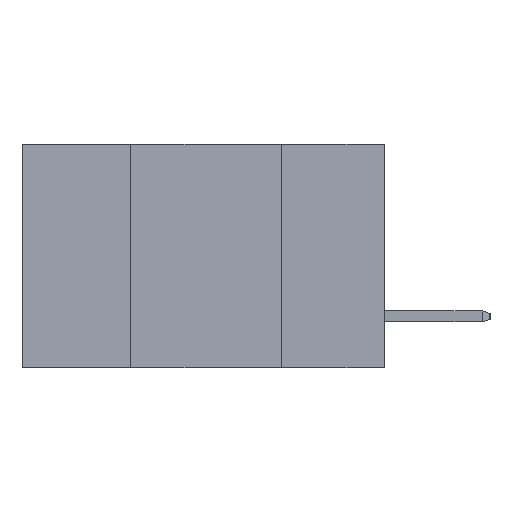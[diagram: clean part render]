
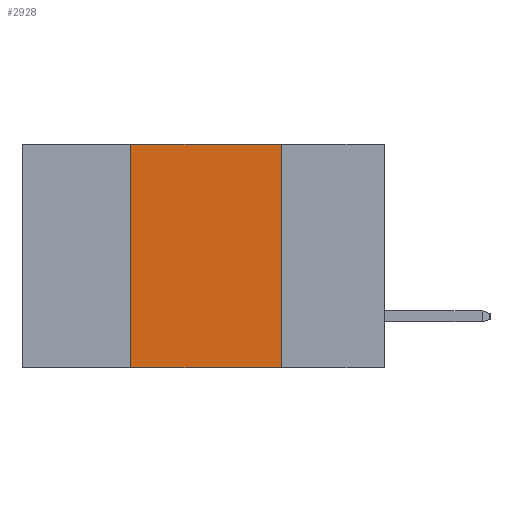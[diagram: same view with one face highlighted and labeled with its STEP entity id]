
A CAD part, left-side view. The second image highlights one B-rep face of the part: STEP entity #2928.
In plain terms, the highlighted planar face has unit normal (-1, 0, 0).
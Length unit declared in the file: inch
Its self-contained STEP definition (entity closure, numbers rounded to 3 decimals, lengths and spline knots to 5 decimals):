
#349 = ORIENTED_EDGE ( 'NONE', *, *, #1069, .F. ) ;
#1027 = LINE ( 'NONE', #5265, #11557 ) ;
#1069 = EDGE_CURVE ( 'NONE', #8265, #10192, #11885, .T. ) ;
#1513 = EDGE_CURVE ( 'NONE', #10192, #11349, #1027, .T. ) ;
#1996 = VECTOR ( 'NONE', #10328, 39.37008 ) ;
#2928 = ADVANCED_FACE ( 'NONE', ( #13454 ), #12463, .F. ) ;
#3131 = VERTEX_POINT ( 'NONE', #9916 ) ;
#3186 = ORIENTED_EDGE ( 'NONE', *, *, #8878, .T. ) ;
#3441 = DIRECTION ( 'NONE',  ( 0., -1., 0. ) ) ;
#3705 = CARTESIAN_POINT ( 'NONE',  ( 0., 0.6, -0.37 ) ) ;
#4680 = LINE ( 'NONE', #3705, #7164 ) ;
#5265 = CARTESIAN_POINT ( 'NONE',  ( 0., 0.6, 0. ) ) ;
#5333 = CARTESIAN_POINT ( 'NONE',  ( 0., 0.42, -0.37 ) ) ;
#5671 = EDGE_LOOP ( 'NONE', ( #10900, #11213, #349, #3186 ) ) ;
#7102 = CARTESIAN_POINT ( 'NONE',  ( 0., 0.42, 0. ) ) ;
#7164 = VECTOR ( 'NONE', #10048, 39.37008 ) ;
#8071 = CARTESIAN_POINT ( 'NONE',  ( 0., 0.42, -0.37 ) ) ;
#8250 = CARTESIAN_POINT ( 'NONE',  ( 0., 0.17, -0.37 ) ) ;
#8265 = VERTEX_POINT ( 'NONE', #8071 ) ;
#8878 = EDGE_CURVE ( 'NONE', #8265, #3131, #4680, .T. ) ;
#9188 = DIRECTION ( 'NONE',  ( 0., 0., 1. ) ) ;
#9442 = CARTESIAN_POINT ( 'NONE',  ( 0., 0.17, 0. ) ) ;
#9916 = CARTESIAN_POINT ( 'NONE',  ( 0., 0.17, -0.37 ) ) ;
#10048 = DIRECTION ( 'NONE',  ( 0., -1., 0. ) ) ;
#10192 = VERTEX_POINT ( 'NONE', #7102 ) ;
#10275 = EDGE_CURVE ( 'NONE', #11349, #3131, #13119, .T. ) ;
#10328 = DIRECTION ( 'NONE',  ( 0., 0., -1. ) ) ;
#10900 = ORIENTED_EDGE ( 'NONE', *, *, #10275, .F. ) ;
#11192 = AXIS2_PLACEMENT_3D ( 'NONE', #12546, #12269, #12252 ) ;
#11213 = ORIENTED_EDGE ( 'NONE', *, *, #1513, .F. ) ;
#11349 = VERTEX_POINT ( 'NONE', #9442 ) ;
#11557 = VECTOR ( 'NONE', #3441, 39.37008 ) ;
#11568 = VECTOR ( 'NONE', #9188, 39.37008 ) ;
#11885 = LINE ( 'NONE', #5333, #11568 ) ;
#12252 = DIRECTION ( 'NONE',  ( 0., 0., -1. ) ) ;
#12269 = DIRECTION ( 'NONE',  ( 1., 0., 0. ) ) ;
#12463 = PLANE ( 'NONE',  #11192 ) ;
#12546 = CARTESIAN_POINT ( 'NONE',  ( 0., 0.6, 0. ) ) ;
#13119 = LINE ( 'NONE', #8250, #1996 ) ;
#13454 = FACE_OUTER_BOUND ( 'NONE', #5671, .T. ) ;
